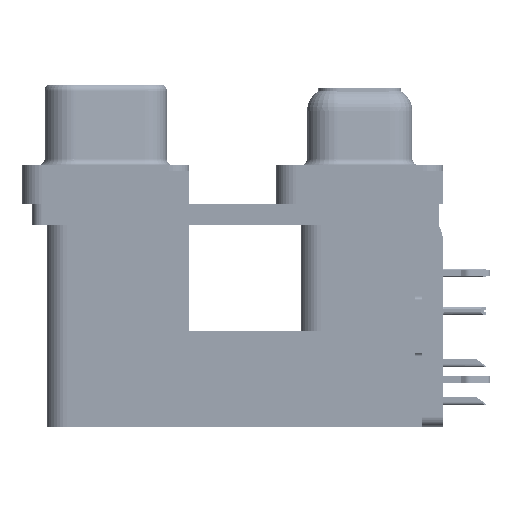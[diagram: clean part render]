
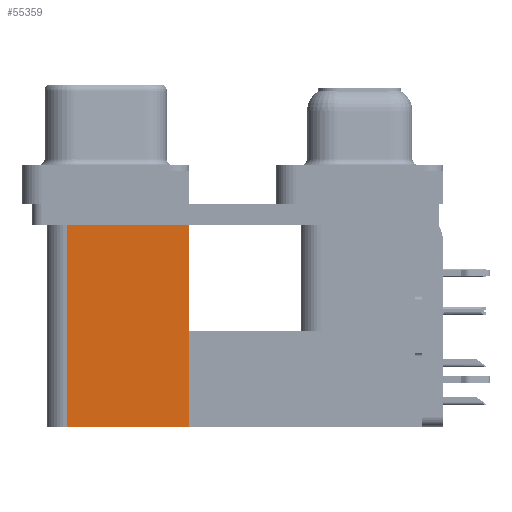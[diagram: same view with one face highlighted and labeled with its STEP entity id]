
A CAD part, left-side view. The second image highlights one B-rep face of the part: STEP entity #55359.
In plain terms, the highlighted planar face has unit normal (-1, 0, 0).
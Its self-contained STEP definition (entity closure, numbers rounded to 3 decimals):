
#666 = ORIENTED_EDGE ( 'NONE', *, *, #44007, .F. ) ;
#1171 = AXIS2_PLACEMENT_3D ( 'NONE', #23136, #22778, #50180 ) ;
#2943 = CARTESIAN_POINT ( 'NONE',  ( 3.79, 12.775, -19.2 ) ) ;
#3272 = CARTESIAN_POINT ( 'NONE',  ( 3.79, 12.775, -19.2 ) ) ;
#4482 = VECTOR ( 'NONE', #68736, 1000. ) ;
#7546 = LINE ( 'NONE', #3272, #55131 ) ;
#8270 = LINE ( 'NONE', #2943, #4482 ) ;
#10792 = EDGE_CURVE ( 'NONE', #18860, #29363, #8270, .T. ) ;
#11110 = DIRECTION ( 'NONE',  ( 0., 1., 0. ) ) ;
#12103 = FACE_OUTER_BOUND ( 'NONE', #19540, .T. ) ;
#15473 = CARTESIAN_POINT ( 'NONE',  ( 3.79, 21.975, -19.2 ) ) ;
#16616 = VERTEX_POINT ( 'NONE', #15473 ) ;
#18860 = VERTEX_POINT ( 'NONE', #69957 ) ;
#19540 = EDGE_LOOP ( 'NONE', ( #51899, #28125, #666, #51299 ) ) ;
#21462 = DIRECTION ( 'NONE',  ( 0., 0., 1. ) ) ;
#22778 = DIRECTION ( 'NONE',  ( 1., 0., 0. ) ) ;
#23136 = CARTESIAN_POINT ( 'NONE',  ( 3.79, 12.775, -19.2 ) ) ;
#24566 = EDGE_CURVE ( 'NONE', #16616, #51600, #64504, .T. ) ;
#27132 = CARTESIAN_POINT ( 'NONE',  ( 3.79, 12.775, -2.5 ) ) ;
#28125 = ORIENTED_EDGE ( 'NONE', *, *, #24566, .F. ) ;
#29251 = DIRECTION ( 'NONE',  ( 0., 1., 0. ) ) ;
#29363 = VERTEX_POINT ( 'NONE', #62722 ) ;
#31911 = EDGE_CURVE ( 'NONE', #29363, #51600, #55219, .T. ) ;
#44007 = EDGE_CURVE ( 'NONE', #18860, #16616, #7546, .T. ) ;
#46206 = VECTOR ( 'NONE', #21462, 1000. ) ;
#48534 = CARTESIAN_POINT ( 'NONE',  ( 3.79, 21.975, -2.5 ) ) ;
#50180 = DIRECTION ( 'NONE',  ( 0., 1., 0. ) ) ;
#51299 = ORIENTED_EDGE ( 'NONE', *, *, #10792, .T. ) ;
#51600 = VERTEX_POINT ( 'NONE', #48534 ) ;
#51899 = ORIENTED_EDGE ( 'NONE', *, *, #31911, .T. ) ;
#55131 = VECTOR ( 'NONE', #29251, 1000. ) ;
#55219 = LINE ( 'NONE', #27132, #58809 ) ;
#55359 = ADVANCED_FACE ( 'NONE', ( #12103 ), #60153, .F. ) ;
#58809 = VECTOR ( 'NONE', #11110, 1000. ) ;
#59176 = CARTESIAN_POINT ( 'NONE',  ( 3.79, 21.975, -19.2 ) ) ;
#60153 = PLANE ( 'NONE',  #1171 ) ;
#62722 = CARTESIAN_POINT ( 'NONE',  ( 3.79, 12.775, -2.5 ) ) ;
#64504 = LINE ( 'NONE', #59176, #46206 ) ;
#68736 = DIRECTION ( 'NONE',  ( 0., 0., 1. ) ) ;
#69957 = CARTESIAN_POINT ( 'NONE',  ( 3.79, 12.775, -19.2 ) ) ;
